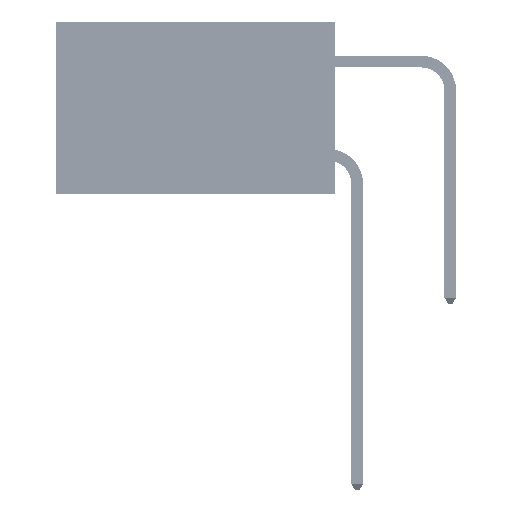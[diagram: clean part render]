
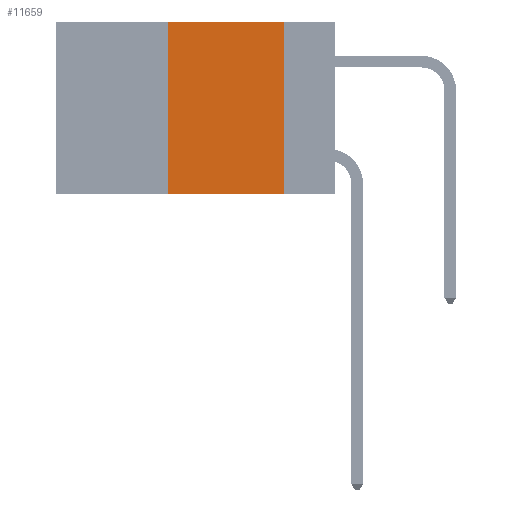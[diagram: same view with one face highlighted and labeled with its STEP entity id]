
A CAD part, left-side view. The second image highlights one B-rep face of the part: STEP entity #11659.
In plain terms, the highlighted planar face has unit normal (-1, 0, 0).
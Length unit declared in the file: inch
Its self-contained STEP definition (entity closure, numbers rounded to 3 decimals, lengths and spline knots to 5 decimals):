
#862 = CARTESIAN_POINT ( 'NONE',  ( 0., 0.36, 0. ) ) ;
#2332 = LINE ( 'NONE', #23888, #23351 ) ;
#3171 = DIRECTION ( 'NONE',  ( 0., -1., 0. ) ) ;
#4624 = ORIENTED_EDGE ( 'NONE', *, *, #42950, .F. ) ;
#7300 = PLANE ( 'NONE',  #19836 ) ;
#8711 = CARTESIAN_POINT ( 'NONE',  ( 0., 0.11, 0. ) ) ;
#10746 = VERTEX_POINT ( 'NONE', #38609 ) ;
#10978 = DIRECTION ( 'NONE',  ( 1., 0., 0. ) ) ;
#11659 = ADVANCED_FACE ( 'NONE', ( #47925 ), #7300, .F. ) ;
#14130 = DIRECTION ( 'NONE',  ( 0., 0., 1. ) ) ;
#17208 = VERTEX_POINT ( 'NONE', #17474 ) ;
#17474 = CARTESIAN_POINT ( 'NONE',  ( 0., 0.11, 0. ) ) ;
#19836 = AXIS2_PLACEMENT_3D ( 'NONE', #19939, #10978, #36609 ) ;
#19892 = EDGE_LOOP ( 'NONE', ( #4624, #29666, #52475, #50188 ) ) ;
#19939 = CARTESIAN_POINT ( 'NONE',  ( 0., 0.6, 0. ) ) ;
#19960 = LINE ( 'NONE', #41877, #29152 ) ;
#23351 = VECTOR ( 'NONE', #3171, 39.37008 ) ;
#23888 = CARTESIAN_POINT ( 'NONE',  ( 0., 0.6, -0.37 ) ) ;
#24403 = EDGE_CURVE ( 'NONE', #31702, #10746, #2332, .T. ) ;
#29152 = VECTOR ( 'NONE', #29571, 39.37008 ) ;
#29571 = DIRECTION ( 'NONE',  ( 0., -1., 0. ) ) ;
#29666 = ORIENTED_EDGE ( 'NONE', *, *, #52820, .F. ) ;
#31702 = VERTEX_POINT ( 'NONE', #43404 ) ;
#34156 = LINE ( 'NONE', #8711, #35487 ) ;
#34955 = EDGE_CURVE ( 'NONE', #31702, #48739, #43714, .T. ) ;
#35487 = VECTOR ( 'NONE', #42250, 39.37008 ) ;
#36609 = DIRECTION ( 'NONE',  ( 0., 0., -1. ) ) ;
#38609 = CARTESIAN_POINT ( 'NONE',  ( 0., 0.11, -0.37 ) ) ;
#41274 = CARTESIAN_POINT ( 'NONE',  ( 0., 0.36, 0. ) ) ;
#41877 = CARTESIAN_POINT ( 'NONE',  ( 0., 0.6, 0. ) ) ;
#42250 = DIRECTION ( 'NONE',  ( 0., 0., -1. ) ) ;
#42403 = VECTOR ( 'NONE', #14130, 39.37008 ) ;
#42950 = EDGE_CURVE ( 'NONE', #17208, #10746, #34156, .T. ) ;
#43404 = CARTESIAN_POINT ( 'NONE',  ( 0., 0.36, -0.37 ) ) ;
#43714 = LINE ( 'NONE', #862, #42403 ) ;
#47925 = FACE_OUTER_BOUND ( 'NONE', #19892, .T. ) ;
#48739 = VERTEX_POINT ( 'NONE', #41274 ) ;
#50188 = ORIENTED_EDGE ( 'NONE', *, *, #24403, .T. ) ;
#52475 = ORIENTED_EDGE ( 'NONE', *, *, #34955, .F. ) ;
#52820 = EDGE_CURVE ( 'NONE', #48739, #17208, #19960, .T. ) ;
